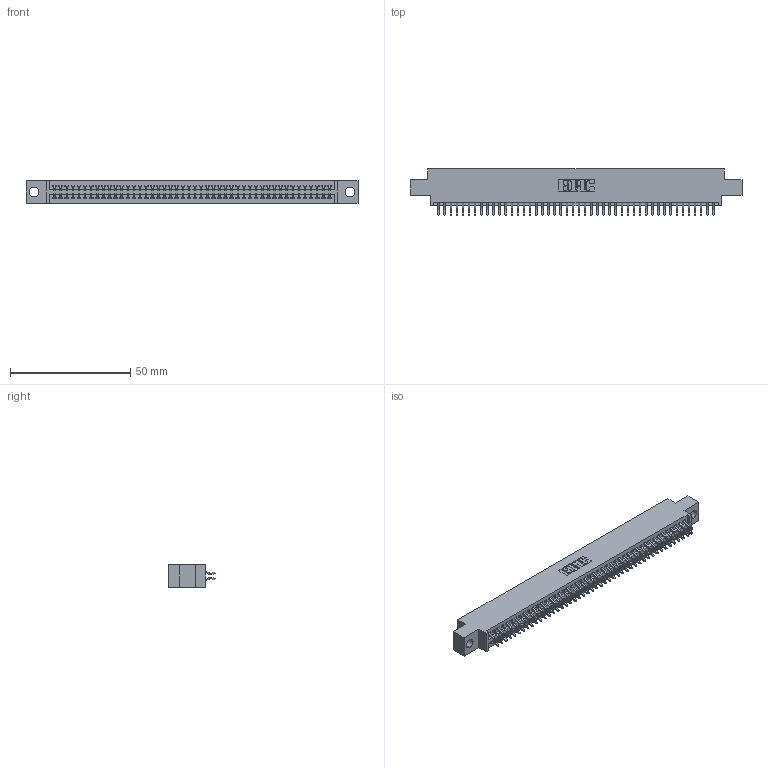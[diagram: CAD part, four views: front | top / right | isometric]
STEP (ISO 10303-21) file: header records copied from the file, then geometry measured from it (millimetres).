
FILE_DESCRIPTION (( 'STEP AP203' ), '1' );
FILE_NAME ('345-092-556-804.STEP', '2021-05-20T15:53:15', ( '' ), ( '' ), 'SwSTEP 2.0', 'SolidWorks 2020', '' );
FILE_SCHEMA (( 'CONFIG_CONTROL_DESIGN' ));
Length unit declared in the file: inch
Products named in the file (3): 345 Part_0.170 Offset - 0.156 Dia-TI; 345-092-556-804; 345-292-001_556 Tail
Assembly tree (93 placements, depth 2):
  345-092-556-804
    345 Part_0.170 Offset - 0.156 Dia-TI
    345-292-001_556 Tail  x92
Bounding box: 138.05 x 19.24 x 9.4 mm (x, y, z)
Volume: 13224.4 mm3; surface area: 19539.8 mm2
Topology: 93 solids, 93 shells, 5296 faces, 15753 edges, 10378 vertices
Faces by surface type: plane 3502, cylinder 1794
Entity records: 36325 total; most frequent: CARTESIAN_POINT 6106, ORIENTED_EDGE 6026, DIRECTION 5365, EDGE_CURVE 3013, VECTOR 2689, LINE 2689, VERTEX_POINT 2006, AXIS2_PLACEMENT_3D 1338
